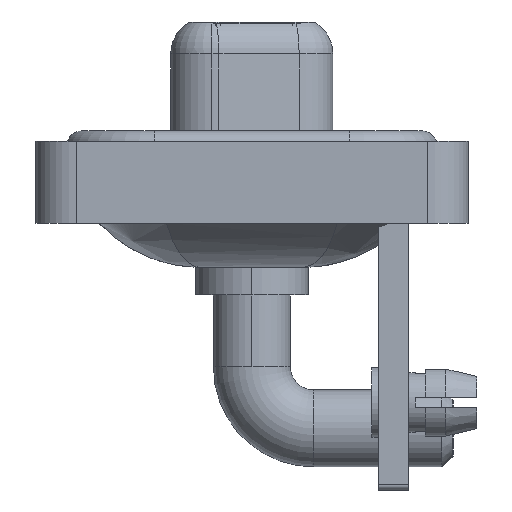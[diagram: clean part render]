
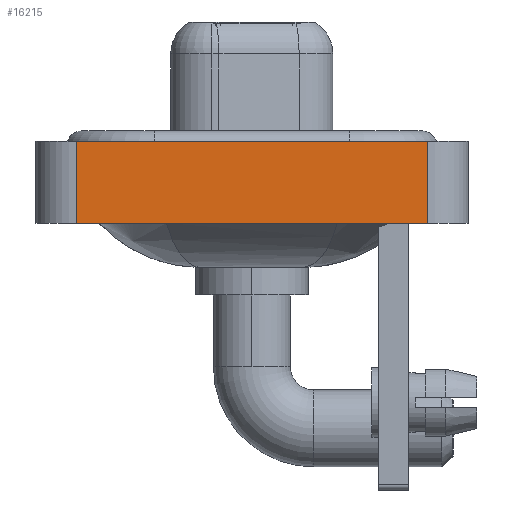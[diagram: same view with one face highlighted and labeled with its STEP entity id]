
A CAD part, left-side view. The second image highlights one B-rep face of the part: STEP entity #16215.
In plain terms, the highlighted planar face has unit normal (-1, 0, 0).
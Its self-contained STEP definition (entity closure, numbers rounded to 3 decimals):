
#986 = EDGE_CURVE ( 'NONE', #3292, #12417, #18964, .T. ) ;
#1609 = DIRECTION ( 'NONE',  ( 0., 0., 1. ) ) ;
#1895 = DIRECTION ( 'NONE',  ( 0., -1., 0. ) ) ;
#2727 = VECTOR ( 'NONE', #7516, 1000. ) ;
#2962 = LINE ( 'NONE', #18216, #19493 ) ;
#3292 = VERTEX_POINT ( 'NONE', #14113 ) ;
#3825 = CARTESIAN_POINT ( 'NONE',  ( -7.3, -8.55, -3.6 ) ) ;
#4177 = DIRECTION ( 'NONE',  ( 0., 0., 1. ) ) ;
#4221 = ORIENTED_EDGE ( 'NONE', *, *, #6431, .T. ) ;
#5147 = FACE_OUTER_BOUND ( 'NONE', #6376, .T. ) ;
#5355 = ORIENTED_EDGE ( 'NONE', *, *, #6664, .F. ) ;
#6166 = VERTEX_POINT ( 'NONE', #3825 ) ;
#6376 = EDGE_LOOP ( 'NONE', ( #4221, #14623, #5355, #12028 ) ) ;
#6431 = EDGE_CURVE ( 'NONE', #6166, #12417, #13737, .T. ) ;
#6551 = CARTESIAN_POINT ( 'NONE',  ( -7.3, -8.55, 0.4 ) ) ;
#6655 = EDGE_CURVE ( 'NONE', #15490, #6166, #16601, .T. ) ;
#6664 = EDGE_CURVE ( 'NONE', #15490, #3292, #2962, .T. ) ;
#6763 = CARTESIAN_POINT ( 'NONE',  ( -7.3, -8.55, -3.6 ) ) ;
#7516 = DIRECTION ( 'NONE',  ( 0., -1., 0. ) ) ;
#8274 = PLANE ( 'NONE',  #15291 ) ;
#10917 = DIRECTION ( 'NONE',  ( 0., 0., 1. ) ) ;
#12028 = ORIENTED_EDGE ( 'NONE', *, *, #6655, .T. ) ;
#12417 = VERTEX_POINT ( 'NONE', #13318 ) ;
#12906 = DIRECTION ( 'NONE',  ( -1., 0., 0. ) ) ;
#13318 = CARTESIAN_POINT ( 'NONE',  ( -7.3, -8.55, 0.4 ) ) ;
#13737 = LINE ( 'NONE', #16965, #16219 ) ;
#14113 = CARTESIAN_POINT ( 'NONE',  ( -7.3, 8.55, 0.4 ) ) ;
#14623 = ORIENTED_EDGE ( 'NONE', *, *, #986, .F. ) ;
#15291 = AXIS2_PLACEMENT_3D ( 'NONE', #6763, #12906, #10917 ) ;
#15490 = VERTEX_POINT ( 'NONE', #18100 ) ;
#16215 = ADVANCED_FACE ( 'NONE', ( #5147 ), #8274, .T. ) ;
#16219 = VECTOR ( 'NONE', #1609, 1000. ) ;
#16497 = CARTESIAN_POINT ( 'NONE',  ( -7.3, -8.55, -3.6 ) ) ;
#16601 = LINE ( 'NONE', #16497, #2727 ) ;
#16965 = CARTESIAN_POINT ( 'NONE',  ( -7.3, -8.55, -3.6 ) ) ;
#17403 = VECTOR ( 'NONE', #1895, 1000. ) ;
#18100 = CARTESIAN_POINT ( 'NONE',  ( -7.3, 8.55, -3.6 ) ) ;
#18216 = CARTESIAN_POINT ( 'NONE',  ( -7.3, 8.55, -3.6 ) ) ;
#18964 = LINE ( 'NONE', #6551, #17403 ) ;
#19493 = VECTOR ( 'NONE', #4177, 1000. ) ;
